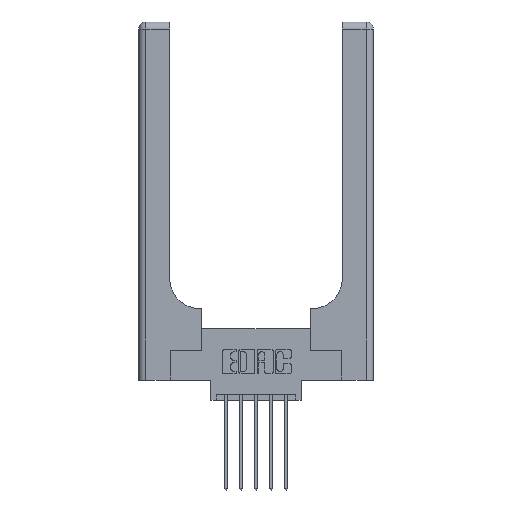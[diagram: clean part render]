
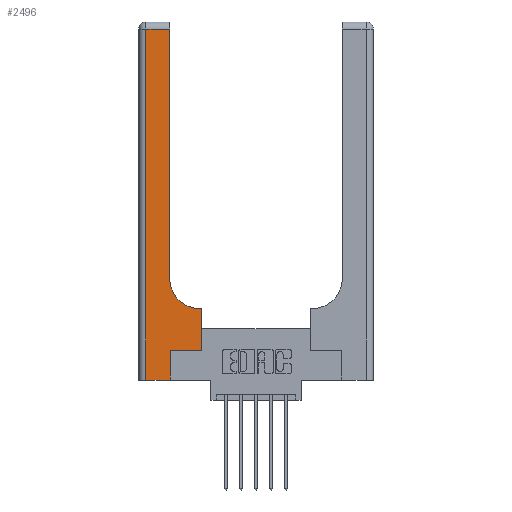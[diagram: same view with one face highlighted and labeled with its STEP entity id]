
A CAD part, top view. The second image highlights one B-rep face of the part: STEP entity #2496.
In plain terms, the highlighted planar face has unit normal (0, 0, 1).
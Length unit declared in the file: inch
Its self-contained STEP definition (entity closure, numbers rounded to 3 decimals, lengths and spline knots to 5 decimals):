
#14 = VECTOR ( 'NONE', #1651, 39.37008 ) ;
#26 = LINE ( 'NONE', #7701, #6942 ) ;
#379 = ORIENTED_EDGE ( 'NONE', *, *, #7438, .T. ) ;
#454 = VECTOR ( 'NONE', #13693, 39.37008 ) ;
#529 = LINE ( 'NONE', #7923, #926 ) ;
#646 = ORIENTED_EDGE ( 'NONE', *, *, #3000, .T. ) ;
#647 = ORIENTED_EDGE ( 'NONE', *, *, #9283, .T. ) ;
#926 = VECTOR ( 'NONE', #2468, 39.37008 ) ;
#1011 = VERTEX_POINT ( 'NONE', #6813 ) ;
#1124 = DIRECTION ( 'NONE',  ( -1., 0., 0. ) ) ;
#1375 = ORIENTED_EDGE ( 'NONE', *, *, #6619, .T. ) ;
#1449 = AXIS2_PLACEMENT_3D ( 'NONE', #2708, #6091, #9199 ) ;
#1651 = DIRECTION ( 'NONE',  ( 1., 0., 0. ) ) ;
#1657 = ORIENTED_EDGE ( 'NONE', *, *, #11554, .T. ) ;
#1659 = CARTESIAN_POINT ( 'NONE',  ( 0.265, 0., 0.37 ) ) ;
#2468 = DIRECTION ( 'NONE',  ( -1., 0., 0. ) ) ;
#2496 = ADVANCED_FACE ( 'NONE', ( #8563 ), #3353, .F. ) ;
#2620 = CARTESIAN_POINT ( 'NONE',  ( 0.26, 2.94, 0.37 ) ) ;
#2708 = CARTESIAN_POINT ( 'NONE',  ( 0.51, 0.85, 0.37 ) ) ;
#3000 = EDGE_CURVE ( 'NONE', #3957, #5706, #26, .T. ) ;
#3038 = VECTOR ( 'NONE', #7531, 39.37008 ) ;
#3353 = PLANE ( 'NONE',  #11708 ) ;
#3513 = VECTOR ( 'NONE', #12225, 39.37008 ) ;
#3957 = VERTEX_POINT ( 'NONE', #6749 ) ;
#3960 = VERTEX_POINT ( 'NONE', #5884 ) ;
#4427 = EDGE_CURVE ( 'NONE', #9555, #7464, #8078, .T. ) ;
#4802 = EDGE_CURVE ( 'NONE', #13577, #11795, #11345, .T. ) ;
#4807 = LINE ( 'NONE', #9118, #3513 ) ;
#4810 = EDGE_CURVE ( 'NONE', #1011, #13577, #4922, .T. ) ;
#4922 = LINE ( 'NONE', #11131, #14 ) ;
#4983 = CARTESIAN_POINT ( 'NONE',  ( 0.26, 0.85, 0.37 ) ) ;
#5650 = CARTESIAN_POINT ( 'NONE',  ( 0.06, 2.94, 0.37 ) ) ;
#5706 = VERTEX_POINT ( 'NONE', #9142 ) ;
#5884 = CARTESIAN_POINT ( 'NONE',  ( 0.51, 0.6, 0.37 ) ) ;
#6091 = DIRECTION ( 'NONE',  ( 0., 0., -1. ) ) ;
#6619 = EDGE_CURVE ( 'NONE', #5706, #1011, #13551, .T. ) ;
#6749 = CARTESIAN_POINT ( 'NONE',  ( 0.06, 0., 0.37 ) ) ;
#6783 = DIRECTION ( 'NONE',  ( 1., 0., 0. ) ) ;
#6813 = CARTESIAN_POINT ( 'NONE',  ( 0.265, 0.25, 0.37 ) ) ;
#6940 = CARTESIAN_POINT ( 'NONE',  ( 0.26, 3., 0.37 ) ) ;
#6942 = VECTOR ( 'NONE', #6783, 39.37008 ) ;
#7039 = CARTESIAN_POINT ( 'NONE',  ( 0.528, 0.25, 0.37 ) ) ;
#7085 = ORIENTED_EDGE ( 'NONE', *, *, #12803, .T. ) ;
#7438 = EDGE_CURVE ( 'NONE', #7464, #11808, #529, .T. ) ;
#7464 = VERTEX_POINT ( 'NONE', #2620 ) ;
#7470 = LINE ( 'NONE', #13775, #3038 ) ;
#7531 = DIRECTION ( 'NONE',  ( -1., 0., 0. ) ) ;
#7555 = CARTESIAN_POINT ( 'NONE',  ( 0.528, 0.6, 0.37 ) ) ;
#7701 = CARTESIAN_POINT ( 'NONE',  ( 0., 0., 0.37 ) ) ;
#7923 = CARTESIAN_POINT ( 'NONE',  ( 0., 2.94, 0.37 ) ) ;
#8078 = LINE ( 'NONE', #6940, #8587 ) ;
#8563 = FACE_OUTER_BOUND ( 'NONE', #10880, .T. ) ;
#8587 = VECTOR ( 'NONE', #13441, 39.37008 ) ;
#8829 = VECTOR ( 'NONE', #13401, 39.37008 ) ;
#9118 = CARTESIAN_POINT ( 'NONE',  ( 0.06, 3., 0.37 ) ) ;
#9142 = CARTESIAN_POINT ( 'NONE',  ( 0.265, 0., 0.37 ) ) ;
#9199 = DIRECTION ( 'NONE',  ( 1., 0., 0. ) ) ;
#9283 = EDGE_CURVE ( 'NONE', #11795, #3960, #7470, .T. ) ;
#9555 = VERTEX_POINT ( 'NONE', #4983 ) ;
#10143 = ORIENTED_EDGE ( 'NONE', *, *, #4427, .T. ) ;
#10880 = EDGE_LOOP ( 'NONE', ( #10143, #379, #1657, #646, #1375, #11118, #13179, #647, #7085 ) ) ;
#10899 = CARTESIAN_POINT ( 'NONE',  ( 0., 3., 0.37 ) ) ;
#11118 = ORIENTED_EDGE ( 'NONE', *, *, #4810, .T. ) ;
#11131 = CARTESIAN_POINT ( 'NONE',  ( 0.265, 0.25, 0.37 ) ) ;
#11345 = LINE ( 'NONE', #7039, #8829 ) ;
#11554 = EDGE_CURVE ( 'NONE', #11808, #3957, #4807, .T. ) ;
#11708 = AXIS2_PLACEMENT_3D ( 'NONE', #10899, #11755, #1124 ) ;
#11755 = DIRECTION ( 'NONE',  ( 0., 0., -1. ) ) ;
#11795 = VERTEX_POINT ( 'NONE', #7555 ) ;
#11808 = VERTEX_POINT ( 'NONE', #5650 ) ;
#12136 = CARTESIAN_POINT ( 'NONE',  ( 0.528, 0.25, 0.37 ) ) ;
#12225 = DIRECTION ( 'NONE',  ( 0., -1., 0. ) ) ;
#12803 = EDGE_CURVE ( 'NONE', #3960, #9555, #13667, .T. ) ;
#13179 = ORIENTED_EDGE ( 'NONE', *, *, #4802, .T. ) ;
#13401 = DIRECTION ( 'NONE',  ( 0., 1., 0. ) ) ;
#13441 = DIRECTION ( 'NONE',  ( 0., 1., 0. ) ) ;
#13551 = LINE ( 'NONE', #1659, #454 ) ;
#13577 = VERTEX_POINT ( 'NONE', #12136 ) ;
#13667 = CIRCLE ( 'NONE', #1449, 0.25 ) ;
#13693 = DIRECTION ( 'NONE',  ( 0., 1., 0. ) ) ;
#13775 = CARTESIAN_POINT ( 'NONE',  ( 0.26, 0.6, 0.37 ) ) ;
